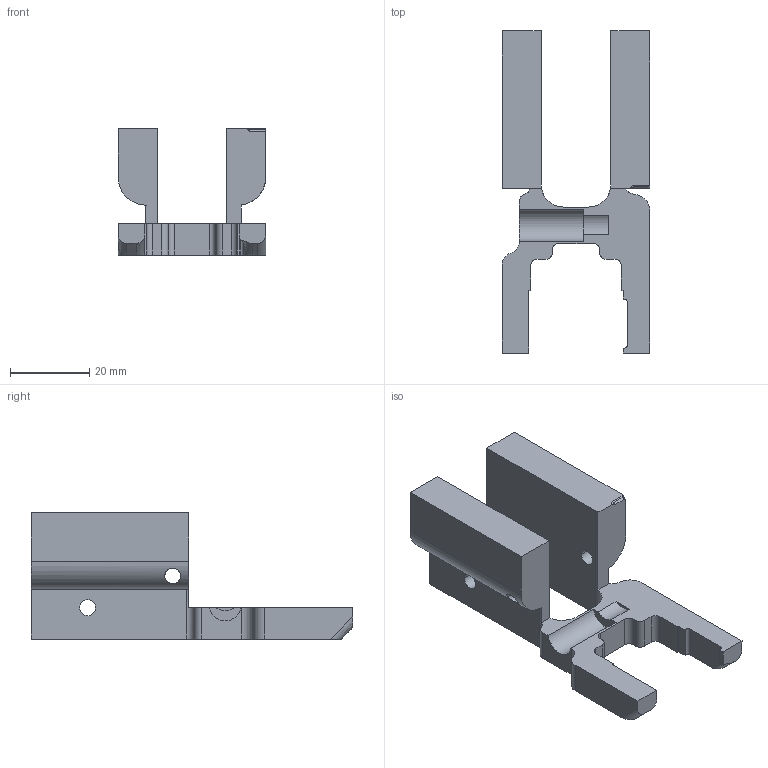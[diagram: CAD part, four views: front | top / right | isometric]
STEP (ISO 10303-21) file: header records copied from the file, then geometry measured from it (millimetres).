
FILE_DESCRIPTION (( 'STEP AP214' ), '1' );
FILE_NAME ('2Fix.STEP', '2013-09-30T13:24:06', ( 'elpi' ), ( '' ), 'SwSTEP 2.0', 'SolidWorks 2013', '' );
FILE_SCHEMA (( 'AUTOMOTIVE_DESIGN' ));
Length unit declared in the file: millimetre
Products named in the file (1): 2Fix
Bounding box: 37.13 x 81.03 x 31.75 mm (x, y, z)
Volume: 22046.1 mm3; surface area: 10514.8 mm2
Topology: 1 solids, 1 shells, 89 faces, 259 edges, 172 vertices
Faces by surface type: plane 41, cylinder 35, bspline 13
Entity records: 4014 total; most frequent: CARTESIAN_POINT 1698, ORIENTED_EDGE 518, DIRECTION 423, EDGE_CURVE 259, VERTEX_POINT 172, VECTOR 149, LINE 149, AXIS2_PLACEMENT_3D 137
